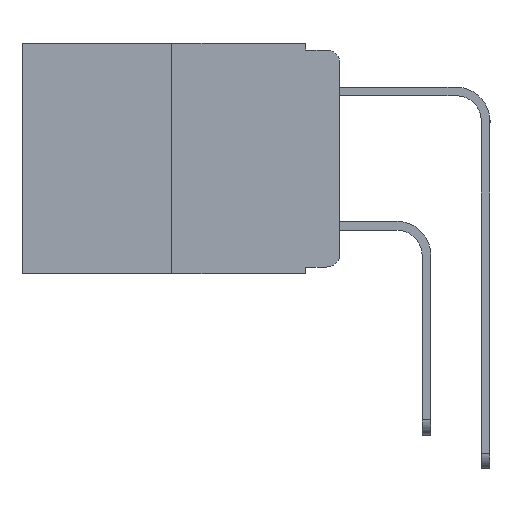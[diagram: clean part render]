
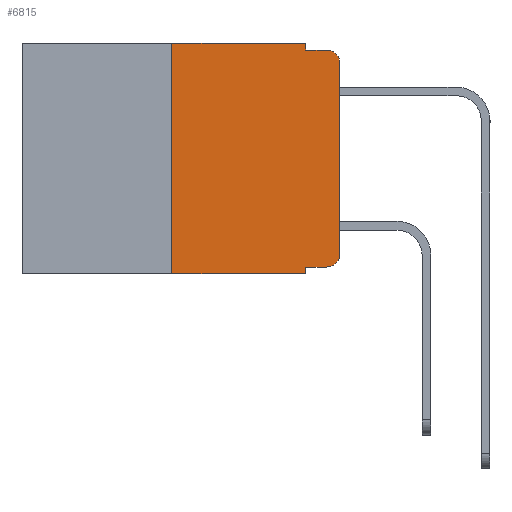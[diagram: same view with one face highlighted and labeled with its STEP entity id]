
A CAD part, left-side view. The second image highlights one B-rep face of the part: STEP entity #6815.
In plain terms, the highlighted planar face has unit normal (-1, 0, 0).
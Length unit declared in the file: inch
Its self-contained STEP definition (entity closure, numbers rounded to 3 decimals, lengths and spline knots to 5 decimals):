
#46 = DIRECTION ( 'NONE',  ( 0., 0., -1. ) ) ;
#61 = ORIENTED_EDGE ( 'NONE', *, *, #12038, .T. ) ;
#173 = ORIENTED_EDGE ( 'NONE', *, *, #11874, .F. ) ;
#250 = CARTESIAN_POINT ( 'NONE',  ( 0., 0.02, -0.333 ) ) ;
#261 = AXIS2_PLACEMENT_3D ( 'NONE', #3590, #11930, #4825 ) ;
#425 = VECTOR ( 'NONE', #4735, 39.37008 ) ;
#548 = ORIENTED_EDGE ( 'NONE', *, *, #11122, .F. ) ;
#666 = CARTESIAN_POINT ( 'NONE',  ( 0., 0.25, 0. ) ) ;
#1250 = VECTOR ( 'NONE', #2067, 39.37008 ) ;
#1402 = VERTEX_POINT ( 'NONE', #4985 ) ;
#1979 = ORIENTED_EDGE ( 'NONE', *, *, #6857, .F. ) ;
#2067 = DIRECTION ( 'NONE',  ( 0., 0., 1. ) ) ;
#2091 = VECTOR ( 'NONE', #6089, 39.37008 ) ;
#2488 = LINE ( 'NONE', #10794, #2091 ) ;
#2588 = CARTESIAN_POINT ( 'NONE',  ( 0., 0.02, -0.313 ) ) ;
#2699 = CARTESIAN_POINT ( 'NONE',  ( 0., 0.051, -0.333 ) ) ;
#3410 = VERTEX_POINT ( 'NONE', #11713 ) ;
#3590 = CARTESIAN_POINT ( 'NONE',  ( 0., 0.02, -0.03 ) ) ;
#3697 = CARTESIAN_POINT ( 'NONE',  ( 0., 0.051, 0. ) ) ;
#3833 = LINE ( 'NONE', #10629, #425 ) ;
#3837 = DIRECTION ( 'NONE',  ( 0., 0., -1. ) ) ;
#3972 = VERTEX_POINT ( 'NONE', #7640 ) ;
#4245 = VERTEX_POINT ( 'NONE', #2699 ) ;
#4351 = VECTOR ( 'NONE', #5967, 39.37008 ) ;
#4497 = VERTEX_POINT ( 'NONE', #4657 ) ;
#4520 = VERTEX_POINT ( 'NONE', #3697 ) ;
#4613 = CARTESIAN_POINT ( 'NONE',  ( 0., 0., 0. ) ) ;
#4657 = CARTESIAN_POINT ( 'NONE',  ( 0., 0.051, -0.343 ) ) ;
#4678 = CARTESIAN_POINT ( 'NONE',  ( 0., 0.473, -0.343 ) ) ;
#4735 = DIRECTION ( 'NONE',  ( 0., 0., -1. ) ) ;
#4825 = DIRECTION ( 'NONE',  ( 0., 0., -1. ) ) ;
#4837 = DIRECTION ( 'NONE',  ( 0., -1., 0. ) ) ;
#4955 = VERTEX_POINT ( 'NONE', #9048 ) ;
#4961 = VERTEX_POINT ( 'NONE', #14642 ) ;
#4985 = CARTESIAN_POINT ( 'NONE',  ( 0., 0.051, -0.01 ) ) ;
#5468 = VECTOR ( 'NONE', #12291, 39.37008 ) ;
#5863 = LINE ( 'NONE', #11177, #5468 ) ;
#5967 = DIRECTION ( 'NONE',  ( 0., -1., 0. ) ) ;
#6089 = DIRECTION ( 'NONE',  ( 0., 0., -1. ) ) ;
#6103 = VECTOR ( 'NONE', #11756, 39.37008 ) ;
#6440 = ORIENTED_EDGE ( 'NONE', *, *, #11951, .T. ) ;
#6450 = EDGE_LOOP ( 'NONE', ( #7696, #7335, #10459, #548, #1979, #12860, #8260, #173, #6440, #61 ) ) ;
#6815 = ADVANCED_FACE ( 'NONE', ( #9424 ), #9732, .F. ) ;
#6857 = EDGE_CURVE ( 'NONE', #9579, #4520, #5863, .T. ) ;
#7335 = ORIENTED_EDGE ( 'NONE', *, *, #7999, .T. ) ;
#7487 = EDGE_CURVE ( 'NONE', #3410, #4497, #13688, .T. ) ;
#7552 = AXIS2_PLACEMENT_3D ( 'NONE', #2588, #11047, #3837 ) ;
#7640 = CARTESIAN_POINT ( 'NONE',  ( 0., 0., -0.03 ) ) ;
#7669 = CARTESIAN_POINT ( 'NONE',  ( 0., 0.051, -0.01 ) ) ;
#7696 = ORIENTED_EDGE ( 'NONE', *, *, #7932, .T. ) ;
#7702 = DIRECTION ( 'NONE',  ( 1., 0., 0. ) ) ;
#7932 = EDGE_CURVE ( 'NONE', #4955, #3972, #9296, .T. ) ;
#7999 = EDGE_CURVE ( 'NONE', #3972, #4961, #10549, .T. ) ;
#8162 = EDGE_CURVE ( 'NONE', #1402, #4961, #11439, .T. ) ;
#8260 = ORIENTED_EDGE ( 'NONE', *, *, #7487, .T. ) ;
#8424 = VECTOR ( 'NONE', #8812, 39.37008 ) ;
#8812 = DIRECTION ( 'NONE',  ( 0., -1., 0. ) ) ;
#9048 = CARTESIAN_POINT ( 'NONE',  ( 0., 0., -0.313 ) ) ;
#9296 = LINE ( 'NONE', #4613, #6103 ) ;
#9424 = FACE_OUTER_BOUND ( 'NONE', #6450, .T. ) ;
#9579 = VERTEX_POINT ( 'NONE', #666 ) ;
#9732 = PLANE ( 'NONE',  #15252 ) ;
#10459 = ORIENTED_EDGE ( 'NONE', *, *, #8162, .F. ) ;
#10549 = CIRCLE ( 'NONE', #261, 0.02 ) ;
#10629 = CARTESIAN_POINT ( 'NONE',  ( 0., 0.051, 0. ) ) ;
#10794 = CARTESIAN_POINT ( 'NONE',  ( 0., 0.051, 0. ) ) ;
#10986 = LINE ( 'NONE', #12814, #1250 ) ;
#11047 = DIRECTION ( 'NONE',  ( -1., 0., 0. ) ) ;
#11122 = EDGE_CURVE ( 'NONE', #4520, #1402, #2488, .T. ) ;
#11177 = CARTESIAN_POINT ( 'NONE',  ( 0., 0.473, 0. ) ) ;
#11439 = LINE ( 'NONE', #7669, #8424 ) ;
#11713 = CARTESIAN_POINT ( 'NONE',  ( 0., 0.25, -0.343 ) ) ;
#11756 = DIRECTION ( 'NONE',  ( 0., 0., 1. ) ) ;
#11774 = EDGE_CURVE ( 'NONE', #3410, #9579, #10986, .T. ) ;
#11874 = EDGE_CURVE ( 'NONE', #4245, #4497, #3833, .T. ) ;
#11930 = DIRECTION ( 'NONE',  ( -1., 0., 0. ) ) ;
#11951 = EDGE_CURVE ( 'NONE', #4245, #12238, #12199, .T. ) ;
#12038 = EDGE_CURVE ( 'NONE', #12238, #4955, #14057, .T. ) ;
#12199 = LINE ( 'NONE', #14122, #15090 ) ;
#12238 = VERTEX_POINT ( 'NONE', #250 ) ;
#12291 = DIRECTION ( 'NONE',  ( 0., -1., 0. ) ) ;
#12814 = CARTESIAN_POINT ( 'NONE',  ( 0., 0.25, 0. ) ) ;
#12860 = ORIENTED_EDGE ( 'NONE', *, *, #11774, .F. ) ;
#13688 = LINE ( 'NONE', #4678, #4351 ) ;
#14057 = CIRCLE ( 'NONE', #7552, 0.02 ) ;
#14122 = CARTESIAN_POINT ( 'NONE',  ( 0., 0.051, -0.333 ) ) ;
#14386 = CARTESIAN_POINT ( 'NONE',  ( 0., 0.473, 0. ) ) ;
#14642 = CARTESIAN_POINT ( 'NONE',  ( 0., 0.02, -0.01 ) ) ;
#15090 = VECTOR ( 'NONE', #4837, 39.37008 ) ;
#15252 = AXIS2_PLACEMENT_3D ( 'NONE', #14386, #7702, #46 ) ;
